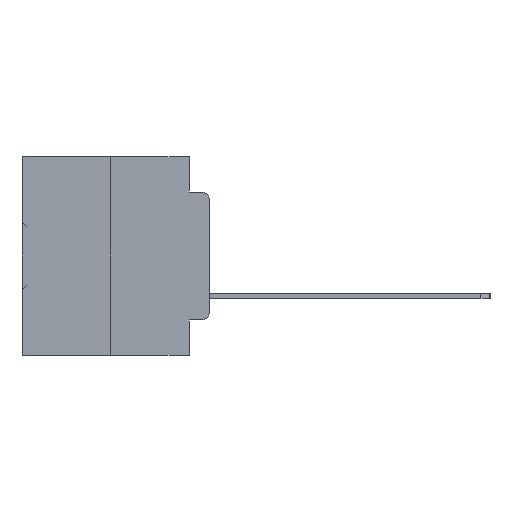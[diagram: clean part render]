
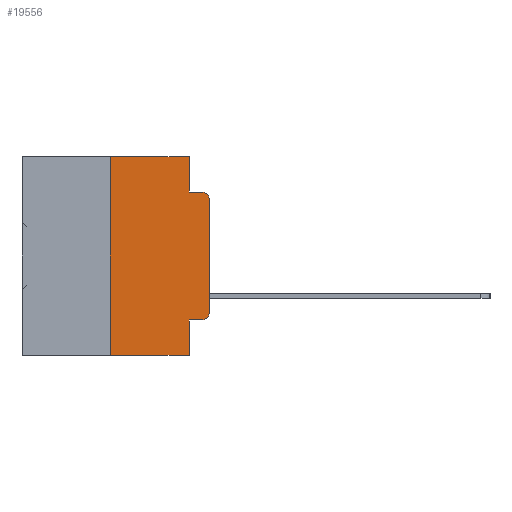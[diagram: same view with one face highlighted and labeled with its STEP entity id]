
A CAD part, left-side view. The second image highlights one B-rep face of the part: STEP entity #19556.
In plain terms, the highlighted planar face has unit normal (-1, 0, 0).
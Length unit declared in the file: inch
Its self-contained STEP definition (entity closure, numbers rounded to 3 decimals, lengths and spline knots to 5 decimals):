
#268 = ORIENTED_EDGE ( 'NONE', *, *, #3410, .F. ) ;
#1089 = DIRECTION ( 'NONE',  ( 1., 0., 0. ) ) ;
#1650 = ORIENTED_EDGE ( 'NONE', *, *, #2290, .T. ) ;
#1677 = CARTESIAN_POINT ( 'NONE',  ( 0., 0.25, 0. ) ) ;
#1690 = ORIENTED_EDGE ( 'NONE', *, *, #3152, .T. ) ;
#1716 = VERTEX_POINT ( 'NONE', #2278 ) ;
#2278 = CARTESIAN_POINT ( 'NONE',  ( 0., 0.051, -0.5 ) ) ;
#2290 = EDGE_CURVE ( 'NONE', #19282, #23825, #10980, .T. ) ;
#2509 = LINE ( 'NONE', #32777, #24483 ) ;
#2676 = CARTESIAN_POINT ( 'NONE',  ( 0., 0., -0.3915 ) ) ;
#2693 = EDGE_CURVE ( 'NONE', #12620, #1716, #5934, .T. ) ;
#2702 = EDGE_CURVE ( 'NONE', #5120, #6426, #13675, .T. ) ;
#3152 = EDGE_CURVE ( 'NONE', #16677, #19282, #21159, .T. ) ;
#3410 = EDGE_CURVE ( 'NONE', #6426, #6220, #12274, .T. ) ;
#3496 = ORIENTED_EDGE ( 'NONE', *, *, #33484, .T. ) ;
#3779 = CARTESIAN_POINT ( 'NONE',  ( 0., 0.02, -0.4115 ) ) ;
#4232 = CARTESIAN_POINT ( 'NONE',  ( 0., 0.051, -0.0885 ) ) ;
#4572 = EDGE_LOOP ( 'NONE', ( #1650, #3496, #35475, #268, #31625, #9831, #17503, #33334, #35916, #1690 ) ) ;
#4686 = AXIS2_PLACEMENT_3D ( 'NONE', #28490, #11509, #31335 ) ;
#5094 = CARTESIAN_POINT ( 'NONE',  ( 0., 0.051, 0. ) ) ;
#5120 = VERTEX_POINT ( 'NONE', #1677 ) ;
#5934 = LINE ( 'NONE', #18703, #28710 ) ;
#6220 = VERTEX_POINT ( 'NONE', #4232 ) ;
#6426 = VERTEX_POINT ( 'NONE', #5094 ) ;
#6587 = VERTEX_POINT ( 'NONE', #23142 ) ;
#6593 = CARTESIAN_POINT ( 'NONE',  ( 0., 0.02, -0.3915 ) ) ;
#8755 = EDGE_CURVE ( 'NONE', #6587, #1716, #35807, .T. ) ;
#9525 = DIRECTION ( 'NONE',  ( 0., 0., -1. ) ) ;
#9831 = ORIENTED_EDGE ( 'NONE', *, *, #28294, .F. ) ;
#10092 = DIRECTION ( 'NONE',  ( 0., -1., 0. ) ) ;
#10702 = CARTESIAN_POINT ( 'NONE',  ( 0., 0.051, -0.4115 ) ) ;
#10946 = CARTESIAN_POINT ( 'NONE',  ( 0., 0.25, 0. ) ) ;
#10980 = LINE ( 'NONE', #19090, #33548 ) ;
#11509 = DIRECTION ( 'NONE',  ( -1., 0., 0. ) ) ;
#12274 = LINE ( 'NONE', #31164, #33897 ) ;
#12531 = CIRCLE ( 'NONE', #4686, 0.02 ) ;
#12620 = VERTEX_POINT ( 'NONE', #26516 ) ;
#12634 = AXIS2_PLACEMENT_3D ( 'NONE', #6593, #26611, #9525 ) ;
#12672 = VECTOR ( 'NONE', #27731, 39.37008 ) ;
#12853 = EDGE_CURVE ( 'NONE', #6587, #16677, #21097, .T. ) ;
#13675 = LINE ( 'NONE', #21540, #20317 ) ;
#15885 = DIRECTION ( 'NONE',  ( 0., -1., 0. ) ) ;
#16677 = VERTEX_POINT ( 'NONE', #3779 ) ;
#17042 = VECTOR ( 'NONE', #27953, 39.37008 ) ;
#17503 = ORIENTED_EDGE ( 'NONE', *, *, #2693, .T. ) ;
#18343 = CARTESIAN_POINT ( 'NONE',  ( 0., 0.051, 0. ) ) ;
#18703 = CARTESIAN_POINT ( 'NONE',  ( 0., 0.473, -0.5 ) ) ;
#19090 = CARTESIAN_POINT ( 'NONE',  ( 0., 0., 0. ) ) ;
#19282 = VERTEX_POINT ( 'NONE', #2676 ) ;
#19556 = ADVANCED_FACE ( 'NONE', ( #21494 ), #35190, .F. ) ;
#19609 = CARTESIAN_POINT ( 'NONE',  ( 0., 0., -0.1085 ) ) ;
#20317 = VECTOR ( 'NONE', #15885, 39.37008 ) ;
#20912 = VECTOR ( 'NONE', #21176, 39.37008 ) ;
#21097 = LINE ( 'NONE', #10702, #12672 ) ;
#21159 = CIRCLE ( 'NONE', #12634, 0.02 ) ;
#21176 = DIRECTION ( 'NONE',  ( 0., 0., -1. ) ) ;
#21213 = DIRECTION ( 'NONE',  ( 0., 0., -1. ) ) ;
#21494 = FACE_OUTER_BOUND ( 'NONE', #4572, .T. ) ;
#21540 = CARTESIAN_POINT ( 'NONE',  ( 0., 0.473, 0. ) ) ;
#23142 = CARTESIAN_POINT ( 'NONE',  ( 0., 0.051, -0.4115 ) ) ;
#23825 = VERTEX_POINT ( 'NONE', #19609 ) ;
#24483 = VECTOR ( 'NONE', #10092, 39.37008 ) ;
#24548 = LINE ( 'NONE', #10946, #17042 ) ;
#26516 = CARTESIAN_POINT ( 'NONE',  ( 0., 0.25, -0.5 ) ) ;
#26611 = DIRECTION ( 'NONE',  ( -1., 0., 0. ) ) ;
#27502 = DIRECTION ( 'NONE',  ( 0., 0., 1. ) ) ;
#27731 = DIRECTION ( 'NONE',  ( 0., -1., 0. ) ) ;
#27953 = DIRECTION ( 'NONE',  ( 0., 0., 1. ) ) ;
#28294 = EDGE_CURVE ( 'NONE', #12620, #5120, #24548, .T. ) ;
#28324 = DIRECTION ( 'NONE',  ( 0., 0., -1. ) ) ;
#28490 = CARTESIAN_POINT ( 'NONE',  ( 0., 0.02, -0.1085 ) ) ;
#28710 = VECTOR ( 'NONE', #35522, 39.37008 ) ;
#29112 = EDGE_CURVE ( 'NONE', #6220, #33011, #2509, .T. ) ;
#31164 = CARTESIAN_POINT ( 'NONE',  ( 0., 0.051, 0. ) ) ;
#31335 = DIRECTION ( 'NONE',  ( 0., 0., -1. ) ) ;
#31625 = ORIENTED_EDGE ( 'NONE', *, *, #2702, .F. ) ;
#31970 = CARTESIAN_POINT ( 'NONE',  ( 0., 0.02, -0.0885 ) ) ;
#32431 = CARTESIAN_POINT ( 'NONE',  ( 0., 0.473, 0. ) ) ;
#32506 = AXIS2_PLACEMENT_3D ( 'NONE', #32431, #1089, #21213 ) ;
#32777 = CARTESIAN_POINT ( 'NONE',  ( 0., 0.051, -0.0885 ) ) ;
#33011 = VERTEX_POINT ( 'NONE', #31970 ) ;
#33334 = ORIENTED_EDGE ( 'NONE', *, *, #8755, .F. ) ;
#33484 = EDGE_CURVE ( 'NONE', #23825, #33011, #12531, .T. ) ;
#33548 = VECTOR ( 'NONE', #27502, 39.37008 ) ;
#33897 = VECTOR ( 'NONE', #28324, 39.37008 ) ;
#35190 = PLANE ( 'NONE',  #32506 ) ;
#35475 = ORIENTED_EDGE ( 'NONE', *, *, #29112, .F. ) ;
#35522 = DIRECTION ( 'NONE',  ( 0., -1., 0. ) ) ;
#35807 = LINE ( 'NONE', #18343, #20912 ) ;
#35916 = ORIENTED_EDGE ( 'NONE', *, *, #12853, .T. ) ;
